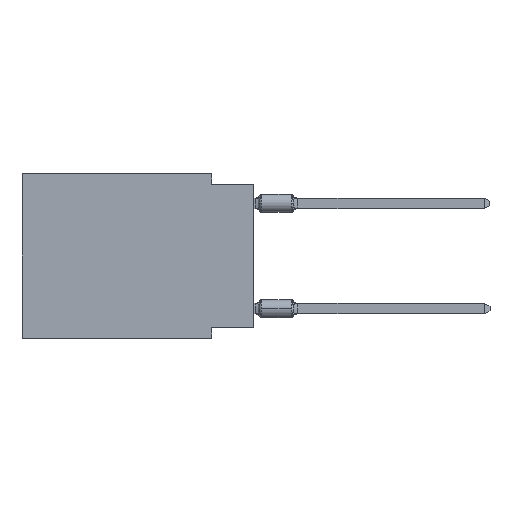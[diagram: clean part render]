
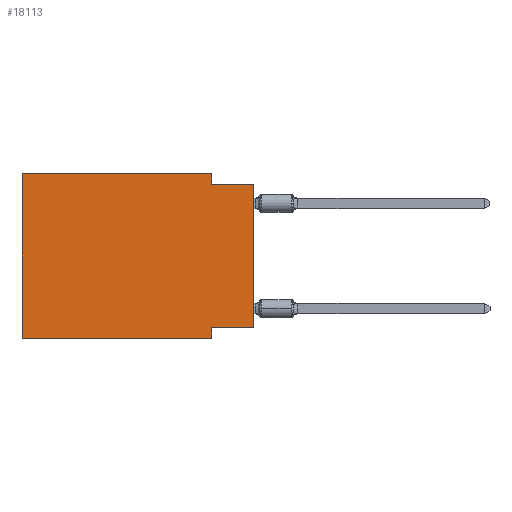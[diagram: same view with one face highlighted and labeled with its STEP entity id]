
A CAD part, left-side view. The second image highlights one B-rep face of the part: STEP entity #18113.
In plain terms, the highlighted planar face has unit normal (-1, 0, 0).
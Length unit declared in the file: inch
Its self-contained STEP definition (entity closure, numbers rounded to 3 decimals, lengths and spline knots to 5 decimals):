
#492 = LINE ( 'NONE', #10761, #2809 ) ;
#542 = LINE ( 'NONE', #10814, #8727 ) ;
#1075 = CARTESIAN_POINT ( 'NONE',  ( 0., 0.1, 0. ) ) ;
#1862 = VERTEX_POINT ( 'NONE', #13072 ) ;
#2038 = CARTESIAN_POINT ( 'NONE',  ( 0., 0., 0. ) ) ;
#2703 = ORIENTED_EDGE ( 'NONE', *, *, #25989, .T. ) ;
#2727 = ORIENTED_EDGE ( 'NONE', *, *, #4357, .F. ) ;
#2809 = VECTOR ( 'NONE', #19076, 39.37008 ) ;
#3254 = LINE ( 'NONE', #5590, #26861 ) ;
#3814 = VERTEX_POINT ( 'NONE', #14930 ) ;
#4000 = ORIENTED_EDGE ( 'NONE', *, *, #8344, .F. ) ;
#4058 = CARTESIAN_POINT ( 'NONE',  ( 0., 0.1, 0. ) ) ;
#4357 = EDGE_CURVE ( 'NONE', #10697, #22521, #542, .T. ) ;
#4731 = CARTESIAN_POINT ( 'NONE',  ( 0., 0.1, -0.39 ) ) ;
#4732 = DIRECTION ( 'NONE',  ( 0., 0., 1. ) ) ;
#5061 = DIRECTION ( 'NONE',  ( 0., 0., -1. ) ) ;
#5590 = CARTESIAN_POINT ( 'NONE',  ( 0., 0.55, -0.39 ) ) ;
#5757 = FACE_OUTER_BOUND ( 'NONE', #24866, .T. ) ;
#7336 = CARTESIAN_POINT ( 'NONE',  ( 0., 0.55, 0. ) ) ;
#7825 = VECTOR ( 'NONE', #19288, 39.37008 ) ;
#8038 = DIRECTION ( 'NONE',  ( 0., 0., -1. ) ) ;
#8112 = VECTOR ( 'NONE', #18436, 39.37008 ) ;
#8344 = EDGE_CURVE ( 'NONE', #3814, #10697, #15063, .T. ) ;
#8727 = VECTOR ( 'NONE', #5061, 39.37008 ) ;
#8949 = VERTEX_POINT ( 'NONE', #15710 ) ;
#9314 = CARTESIAN_POINT ( 'NONE',  ( 0., 0., -0.365 ) ) ;
#9347 = VECTOR ( 'NONE', #4732, 39.37008 ) ;
#9806 = VECTOR ( 'NONE', #20035, 39.37008 ) ;
#10119 = LINE ( 'NONE', #2038, #8112 ) ;
#10697 = VERTEX_POINT ( 'NONE', #14548 ) ;
#10761 = CARTESIAN_POINT ( 'NONE',  ( 0., 0., -0.025 ) ) ;
#10814 = CARTESIAN_POINT ( 'NONE',  ( 0., 0.1, -0.39 ) ) ;
#11700 = CARTESIAN_POINT ( 'NONE',  ( 0., 0.55, 0. ) ) ;
#12017 = VERTEX_POINT ( 'NONE', #1075 ) ;
#12040 = CARTESIAN_POINT ( 'NONE',  ( 0., 0.55, 0. ) ) ;
#12081 = EDGE_CURVE ( 'NONE', #12017, #1862, #22646, .T. ) ;
#13072 = CARTESIAN_POINT ( 'NONE',  ( 0., 0.1, -0.025 ) ) ;
#13342 = LINE ( 'NONE', #7336, #9347 ) ;
#14548 = CARTESIAN_POINT ( 'NONE',  ( 0., 0.1, -0.365 ) ) ;
#14930 = CARTESIAN_POINT ( 'NONE',  ( 0., 0., -0.365 ) ) ;
#15063 = LINE ( 'NONE', #9314, #7825 ) ;
#15098 = VERTEX_POINT ( 'NONE', #19201 ) ;
#15192 = CARTESIAN_POINT ( 'NONE',  ( 0., 0.55, -0.39 ) ) ;
#15482 = VECTOR ( 'NONE', #8038, 39.37008 ) ;
#15710 = CARTESIAN_POINT ( 'NONE',  ( 0., 0.55, 0. ) ) ;
#16679 = ORIENTED_EDGE ( 'NONE', *, *, #12081, .F. ) ;
#16840 = ORIENTED_EDGE ( 'NONE', *, *, #18727, .F. ) ;
#17230 = EDGE_CURVE ( 'NONE', #8949, #12017, #22066, .T. ) ;
#17886 = VERTEX_POINT ( 'NONE', #15192 ) ;
#18113 = ADVANCED_FACE ( 'NONE', ( #5757 ), #26750, .F. ) ;
#18436 = DIRECTION ( 'NONE',  ( 0., 0., 1. ) ) ;
#18701 = DIRECTION ( 'NONE',  ( 0., 0., -1. ) ) ;
#18727 = EDGE_CURVE ( 'NONE', #1862, #15098, #492, .T. ) ;
#18862 = EDGE_CURVE ( 'NONE', #17886, #8949, #13342, .T. ) ;
#19076 = DIRECTION ( 'NONE',  ( 0., -1., 0. ) ) ;
#19201 = CARTESIAN_POINT ( 'NONE',  ( 0., 0., -0.025 ) ) ;
#19288 = DIRECTION ( 'NONE',  ( 0., 1., 0. ) ) ;
#20035 = DIRECTION ( 'NONE',  ( 0., -1., 0. ) ) ;
#20221 = ORIENTED_EDGE ( 'NONE', *, *, #17230, .F. ) ;
#20856 = ORIENTED_EDGE ( 'NONE', *, *, #25713, .T. ) ;
#22066 = LINE ( 'NONE', #11700, #9806 ) ;
#22521 = VERTEX_POINT ( 'NONE', #4731 ) ;
#22646 = LINE ( 'NONE', #4058, #15482 ) ;
#22668 = DIRECTION ( 'NONE',  ( 1., 0., 0. ) ) ;
#23263 = AXIS2_PLACEMENT_3D ( 'NONE', #12040, #22668, #18701 ) ;
#24127 = DIRECTION ( 'NONE',  ( 0., -1., 0. ) ) ;
#24866 = EDGE_LOOP ( 'NONE', ( #20856, #16840, #16679, #20221, #26258, #2703, #2727, #4000 ) ) ;
#25713 = EDGE_CURVE ( 'NONE', #3814, #15098, #10119, .T. ) ;
#25989 = EDGE_CURVE ( 'NONE', #17886, #22521, #3254, .T. ) ;
#26258 = ORIENTED_EDGE ( 'NONE', *, *, #18862, .F. ) ;
#26750 = PLANE ( 'NONE',  #23263 ) ;
#26861 = VECTOR ( 'NONE', #24127, 39.37008 ) ;
